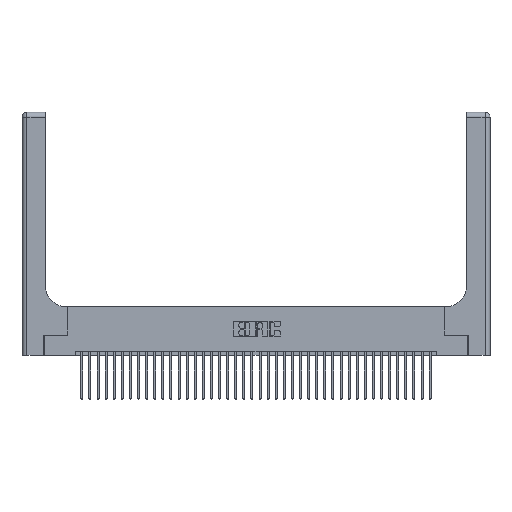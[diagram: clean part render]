
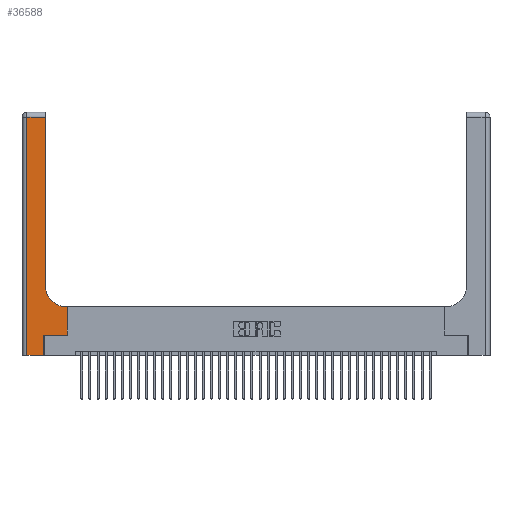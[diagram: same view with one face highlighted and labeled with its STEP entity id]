
A CAD part, top view. The second image highlights one B-rep face of the part: STEP entity #36588.
In plain terms, the highlighted planar face has unit normal (0, 0, 1).
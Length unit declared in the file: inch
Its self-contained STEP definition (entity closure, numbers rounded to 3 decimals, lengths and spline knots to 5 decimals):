
#109 = CARTESIAN_POINT ( 'NONE',  ( 0.5585, 0.25, 0.37 ) ) ;
#176 = CARTESIAN_POINT ( 'NONE',  ( 0.06, 3., 0.37 ) ) ;
#718 = EDGE_CURVE ( 'NONE', #19012, #1322, #24402, .T. ) ;
#855 = VECTOR ( 'NONE', #19553, 39.37008 ) ;
#1143 = VECTOR ( 'NONE', #16927, 39.37008 ) ;
#1322 = VERTEX_POINT ( 'NONE', #10968 ) ;
#1802 = VECTOR ( 'NONE', #24518, 39.37008 ) ;
#2232 = VERTEX_POINT ( 'NONE', #36140 ) ;
#2310 = EDGE_CURVE ( 'NONE', #24843, #2232, #34289, .T. ) ;
#4551 = LINE ( 'NONE', #18274, #28389 ) ;
#5358 = EDGE_CURVE ( 'NONE', #14450, #10926, #28038, .T. ) ;
#6147 = VECTOR ( 'NONE', #38620, 39.37008 ) ;
#6284 = ORIENTED_EDGE ( 'NONE', *, *, #2310, .T. ) ;
#6402 = VERTEX_POINT ( 'NONE', #32904 ) ;
#7577 = ORIENTED_EDGE ( 'NONE', *, *, #5358, .T. ) ;
#8597 = DIRECTION ( 'NONE',  ( 0., 0., -1. ) ) ;
#8802 = DIRECTION ( 'NONE',  ( 1., 0., 0. ) ) ;
#8967 = DIRECTION ( 'NONE',  ( 0., 1., 0. ) ) ;
#9224 = CARTESIAN_POINT ( 'NONE',  ( 0.269, 0., 0.37 ) ) ;
#9284 = CIRCLE ( 'NONE', #36678, 0.25 ) ;
#9449 = VERTEX_POINT ( 'NONE', #16393 ) ;
#10926 = VERTEX_POINT ( 'NONE', #31888 ) ;
#10968 = CARTESIAN_POINT ( 'NONE',  ( 0.2915, 2.94, 0.37 ) ) ;
#11268 = ORIENTED_EDGE ( 'NONE', *, *, #29775, .T. ) ;
#11411 = LINE ( 'NONE', #29391, #6147 ) ;
#13831 = VECTOR ( 'NONE', #27761, 39.37008 ) ;
#14450 = VERTEX_POINT ( 'NONE', #24380 ) ;
#14695 = EDGE_CURVE ( 'NONE', #1322, #14450, #17909, .T. ) ;
#14956 = ORIENTED_EDGE ( 'NONE', *, *, #14695, .T. ) ;
#16284 = FACE_OUTER_BOUND ( 'NONE', #27944, .T. ) ;
#16393 = CARTESIAN_POINT ( 'NONE',  ( 0.5585, 0.25, 0.37 ) ) ;
#16927 = DIRECTION ( 'NONE',  ( -1., 0., 0. ) ) ;
#17289 = CARTESIAN_POINT ( 'NONE',  ( 0.2915, 3., 0.37 ) ) ;
#17909 = LINE ( 'NONE', #25957, #1143 ) ;
#18274 = CARTESIAN_POINT ( 'NONE',  ( 0., 0., 0.37 ) ) ;
#19012 = VERTEX_POINT ( 'NONE', #37454 ) ;
#19254 = ORIENTED_EDGE ( 'NONE', *, *, #23751, .T. ) ;
#19553 = DIRECTION ( 'NONE',  ( 1., 0., 0. ) ) ;
#21549 = VECTOR ( 'NONE', #29752, 39.37008 ) ;
#21998 = CARTESIAN_POINT ( 'NONE',  ( 0.5415, 0.6, 0.37 ) ) ;
#22494 = EDGE_CURVE ( 'NONE', #9449, #6402, #38526, .T. ) ;
#23751 = EDGE_CURVE ( 'NONE', #10926, #24843, #4551, .T. ) ;
#23899 = DIRECTION ( 'NONE',  ( 0., 0., -1. ) ) ;
#24380 = CARTESIAN_POINT ( 'NONE',  ( 0.06, 2.94, 0.37 ) ) ;
#24402 = LINE ( 'NONE', #17289, #21549 ) ;
#24518 = DIRECTION ( 'NONE',  ( 0., 1., 0. ) ) ;
#24843 = VERTEX_POINT ( 'NONE', #29609 ) ;
#24878 = ORIENTED_EDGE ( 'NONE', *, *, #718, .T. ) ;
#24931 = EDGE_CURVE ( 'NONE', #32247, #19012, #9284, .T. ) ;
#25957 = CARTESIAN_POINT ( 'NONE',  ( 0., 2.94, 0.37 ) ) ;
#26830 = DIRECTION ( 'NONE',  ( 1., 0., 0. ) ) ;
#27081 = CARTESIAN_POINT ( 'NONE',  ( 0.5415, 0.85, 0.37 ) ) ;
#27761 = DIRECTION ( 'NONE',  ( 0., -1., 0. ) ) ;
#27944 = EDGE_LOOP ( 'NONE', ( #24878, #14956, #7577, #19254, #6284, #11268, #27998, #37582, #36919 ) ) ;
#27998 = ORIENTED_EDGE ( 'NONE', *, *, #22494, .T. ) ;
#28038 = LINE ( 'NONE', #176, #13831 ) ;
#28389 = VECTOR ( 'NONE', #8802, 39.37008 ) ;
#29391 = CARTESIAN_POINT ( 'NONE',  ( 0.2915, 0.6, 0.37 ) ) ;
#29609 = CARTESIAN_POINT ( 'NONE',  ( 0.269, 0., 0.37 ) ) ;
#29632 = CARTESIAN_POINT ( 'NONE',  ( 0., 3., 0.37 ) ) ;
#29688 = AXIS2_PLACEMENT_3D ( 'NONE', #29632, #8597, #35779 ) ;
#29752 = DIRECTION ( 'NONE',  ( 0., 1., 0. ) ) ;
#29775 = EDGE_CURVE ( 'NONE', #2232, #9449, #33305, .T. ) ;
#31888 = CARTESIAN_POINT ( 'NONE',  ( 0.06, 0., 0.37 ) ) ;
#31896 = VECTOR ( 'NONE', #8967, 39.37008 ) ;
#32247 = VERTEX_POINT ( 'NONE', #21998 ) ;
#32904 = CARTESIAN_POINT ( 'NONE',  ( 0.5585, 0.6, 0.37 ) ) ;
#32972 = PLANE ( 'NONE',  #29688 ) ;
#33305 = LINE ( 'NONE', #38196, #855 ) ;
#34289 = LINE ( 'NONE', #9224, #31896 ) ;
#35779 = DIRECTION ( 'NONE',  ( -1., 0., 0. ) ) ;
#36140 = CARTESIAN_POINT ( 'NONE',  ( 0.269, 0.25, 0.37 ) ) ;
#36588 = ADVANCED_FACE ( 'NONE', ( #16284 ), #32972, .F. ) ;
#36678 = AXIS2_PLACEMENT_3D ( 'NONE', #27081, #23899, #26830 ) ;
#36919 = ORIENTED_EDGE ( 'NONE', *, *, #24931, .T. ) ;
#37454 = CARTESIAN_POINT ( 'NONE',  ( 0.2915, 0.85, 0.37 ) ) ;
#37582 = ORIENTED_EDGE ( 'NONE', *, *, #37851, .T. ) ;
#37851 = EDGE_CURVE ( 'NONE', #6402, #32247, #11411, .T. ) ;
#38196 = CARTESIAN_POINT ( 'NONE',  ( 0.269, 0.25, 0.37 ) ) ;
#38526 = LINE ( 'NONE', #109, #1802 ) ;
#38620 = DIRECTION ( 'NONE',  ( -1., 0., 0. ) ) ;
